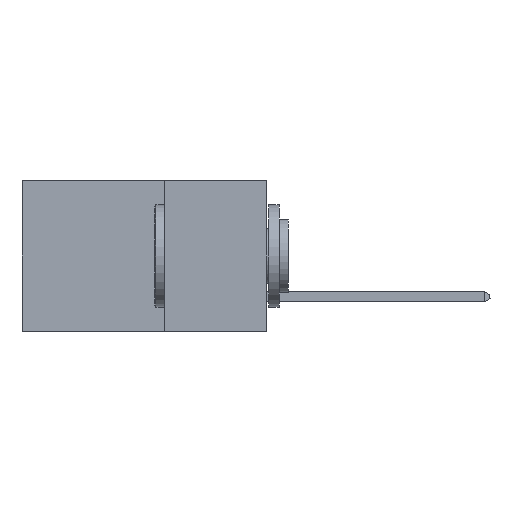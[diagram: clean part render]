
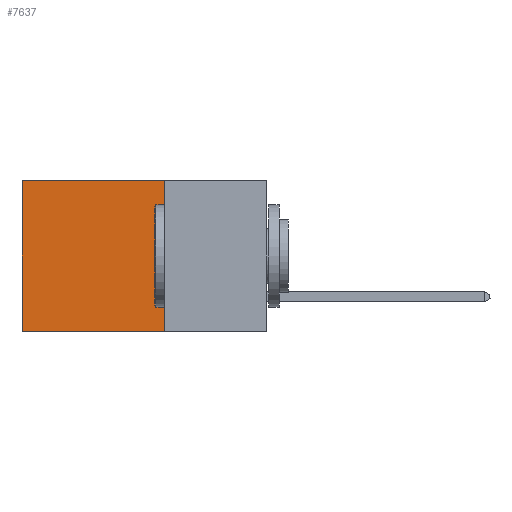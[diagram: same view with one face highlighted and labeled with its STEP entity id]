
A CAD part, left-side view. The second image highlights one B-rep face of the part: STEP entity #7637.
In plain terms, the highlighted planar face has unit normal (-1, 0, 0).
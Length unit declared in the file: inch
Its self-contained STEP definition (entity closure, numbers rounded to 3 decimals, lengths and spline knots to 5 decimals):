
#95 = VERTEX_POINT ( 'NONE', #7230 ) ;
#158 = VERTEX_POINT ( 'NONE', #2831 ) ;
#248 = ORIENTED_EDGE ( 'NONE', *, *, #11456, .F. ) ;
#1153 = ORIENTED_EDGE ( 'NONE', *, *, #4589, .T. ) ;
#1574 = DIRECTION ( 'NONE',  ( 0., 0., -1. ) ) ;
#2547 = DIRECTION ( 'NONE',  ( 0., 0., -1. ) ) ;
#2568 = FACE_OUTER_BOUND ( 'NONE', #13049, .T. ) ;
#2831 = CARTESIAN_POINT ( 'NONE',  ( 0.2875, 0.6, 0. ) ) ;
#3505 = LINE ( 'NONE', #14636, #6235 ) ;
#3683 = ORIENTED_EDGE ( 'NONE', *, *, #12957, .F. ) ;
#3850 = LINE ( 'NONE', #7393, #6549 ) ;
#4041 = DIRECTION ( 'NONE',  ( 0., 1., 0. ) ) ;
#4204 = CARTESIAN_POINT ( 'NONE',  ( 0.2875, 0.25, 0. ) ) ;
#4245 = DIRECTION ( 'NONE',  ( 1., 0., 0. ) ) ;
#4408 = VERTEX_POINT ( 'NONE', #5648 ) ;
#4580 = LINE ( 'NONE', #8328, #10374 ) ;
#4589 = EDGE_CURVE ( 'NONE', #95, #158, #5085, .T. ) ;
#5085 = LINE ( 'NONE', #4204, #7780 ) ;
#5648 = CARTESIAN_POINT ( 'NONE',  ( 0.2875, 0.6, -0.37 ) ) ;
#6235 = VECTOR ( 'NONE', #12439, 39.37008 ) ;
#6549 = VECTOR ( 'NONE', #1574, 39.37008 ) ;
#7230 = CARTESIAN_POINT ( 'NONE',  ( 0.2875, 0.25, 0. ) ) ;
#7393 = CARTESIAN_POINT ( 'NONE',  ( 0.2875, 0.6, 0. ) ) ;
#7637 = ADVANCED_FACE ( 'NONE', ( #2568 ), #11184, .F. ) ;
#7662 = CARTESIAN_POINT ( 'NONE',  ( 0.2875, 0.25, 0. ) ) ;
#7780 = VECTOR ( 'NONE', #4041, 39.37008 ) ;
#8328 = CARTESIAN_POINT ( 'NONE',  ( 0.2875, 0.25, 0. ) ) ;
#8586 = ORIENTED_EDGE ( 'NONE', *, *, #8642, .T. ) ;
#8642 = EDGE_CURVE ( 'NONE', #158, #4408, #3850, .T. ) ;
#10374 = VECTOR ( 'NONE', #2547, 39.37008 ) ;
#11184 = PLANE ( 'NONE',  #14064 ) ;
#11332 = VERTEX_POINT ( 'NONE', #13376 ) ;
#11456 = EDGE_CURVE ( 'NONE', #11332, #4408, #3505, .T. ) ;
#12381 = DIRECTION ( 'NONE',  ( 0., 0., -1. ) ) ;
#12439 = DIRECTION ( 'NONE',  ( 0., 1., 0. ) ) ;
#12957 = EDGE_CURVE ( 'NONE', #95, #11332, #4580, .T. ) ;
#13049 = EDGE_LOOP ( 'NONE', ( #8586, #248, #3683, #1153 ) ) ;
#13376 = CARTESIAN_POINT ( 'NONE',  ( 0.2875, 0.25, -0.37 ) ) ;
#14064 = AXIS2_PLACEMENT_3D ( 'NONE', #7662, #4245, #12381 ) ;
#14636 = CARTESIAN_POINT ( 'NONE',  ( 0.2875, 0.25, -0.37 ) ) ;
